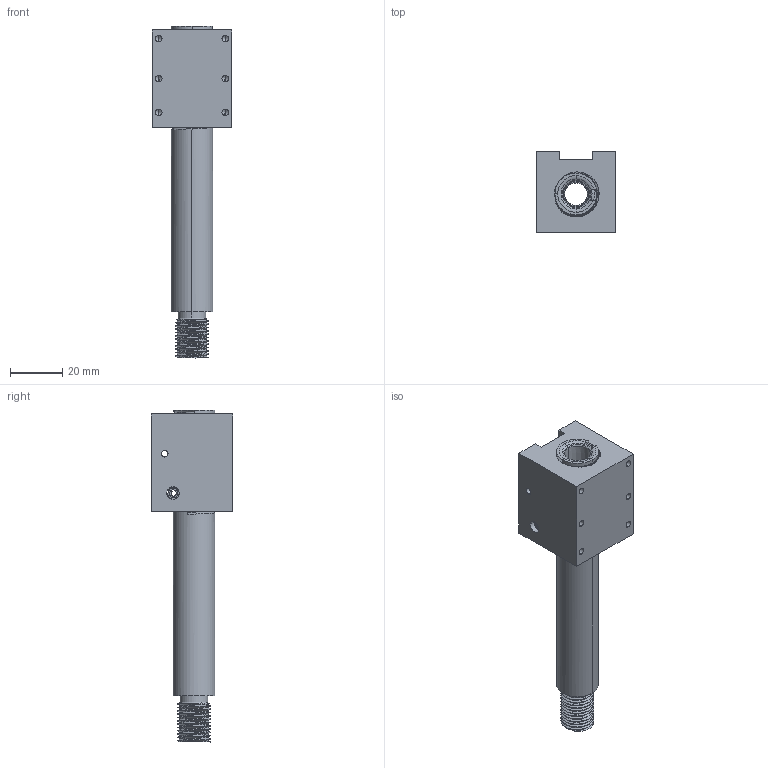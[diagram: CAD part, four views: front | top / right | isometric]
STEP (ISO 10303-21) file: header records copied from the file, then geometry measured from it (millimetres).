
FILE_DESCRIPTION (( 'STEP AP214' ), '1' );
FILE_NAME ('PPDW9 Modcat ECM Barrel and block.STEP', '2020-12-29T21:19:43', ( '' ), ( '' ), 'SwSTEP 2.0', 'SolidWorks 2020', '' );
FILE_SCHEMA (( 'AUTOMOTIVE_DESIGN' ));
Length unit declared in the file: inch
Products named in the file (4): Barrel PPDW9  V3 ECM barrel; PPDW9 Modcat ECM Barrel and block; Barrel block ECM; Barrel spring pin 95755A324_95755A324
Assembly tree (3 placements, depth 2):
  PPDW9 Modcat ECM Barrel and block
    Barrel block ECM
    Barrel PPDW9  V3 ECM barrel
    Barrel spring pin 95755A324_95755A324
Bounding box: 30.48 x 31.24 x 126.82 mm (x, y, z)
Volume: 39998.8 mm3; surface area: 22876.4 mm2
Topology: 3 solids, 3 shells, 229 faces, 654 edges, 424 vertices
Faces by surface type: cylinder 151, plane 26, cone 24, bspline 24, torus 4
Entity records: 31877 total; most frequent: CARTESIAN_POINT 26479, ORIENTED_EDGE 1284, DIRECTION 841, EDGE_CURVE 642, VERTEX_POINT 424, AXIS2_PLACEMENT_3D 316, EDGE_LOOP 244, ADVANCED_FACE 229
